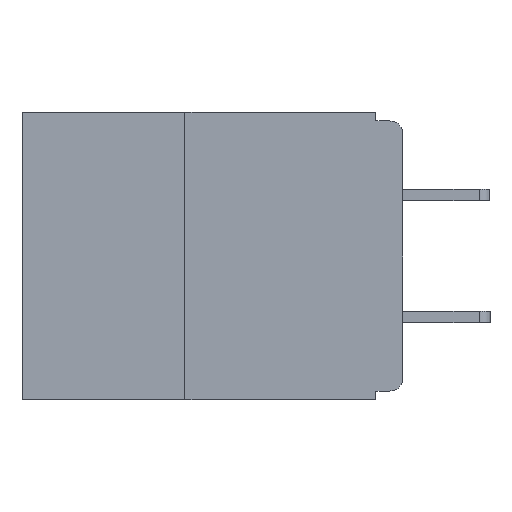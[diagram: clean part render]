
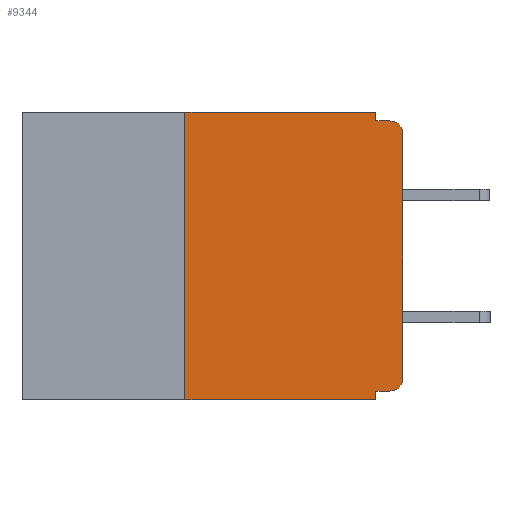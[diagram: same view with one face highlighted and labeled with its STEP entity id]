
A CAD part, left-side view. The second image highlights one B-rep face of the part: STEP entity #9344.
In plain terms, the highlighted planar face has unit normal (-1, 0, 0).
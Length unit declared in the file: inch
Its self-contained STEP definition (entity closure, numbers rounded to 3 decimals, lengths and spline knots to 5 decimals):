
#28 = CARTESIAN_POINT ( 'NONE',  ( 0., 0.031, -0.01 ) ) ;
#310 = VERTEX_POINT ( 'NONE', #12616 ) ;
#390 = CARTESIAN_POINT ( 'NONE',  ( 0., 0.437, -0.33 ) ) ;
#530 = CARTESIAN_POINT ( 'NONE',  ( 0., 0.015, -0.01 ) ) ;
#1196 = LINE ( 'NONE', #18396, #6299 ) ;
#1780 = VERTEX_POINT ( 'NONE', #16016 ) ;
#1913 = LINE ( 'NONE', #8565, #17554 ) ;
#2015 = VECTOR ( 'NONE', #24673, 39.37008 ) ;
#2554 = DIRECTION ( 'NONE',  ( 0., 1., 0. ) ) ;
#2694 = DIRECTION ( 'NONE',  ( 0., 0., -1. ) ) ;
#2735 = CARTESIAN_POINT ( 'NONE',  ( 0., 0.031, 0. ) ) ;
#2963 = DIRECTION ( 'NONE',  ( 0., 0., 1. ) ) ;
#4856 = VERTEX_POINT ( 'NONE', #12094 ) ;
#5527 = EDGE_CURVE ( 'NONE', #16227, #8673, #24029, .T. ) ;
#5559 = ORIENTED_EDGE ( 'NONE', *, *, #15498, .T. ) ;
#5974 = ORIENTED_EDGE ( 'NONE', *, *, #18405, .F. ) ;
#6143 = EDGE_CURVE ( 'NONE', #23200, #10950, #21404, .T. ) ;
#6175 = ORIENTED_EDGE ( 'NONE', *, *, #25741, .F. ) ;
#6299 = VECTOR ( 'NONE', #7874, 39.37008 ) ;
#7097 = AXIS2_PLACEMENT_3D ( 'NONE', #14998, #14834, #14744 ) ;
#7189 = DIRECTION ( 'NONE',  ( 0., 0., -1. ) ) ;
#7194 = DIRECTION ( 'NONE',  ( 1., 0., 0. ) ) ;
#7321 = PLANE ( 'NONE',  #12634 ) ;
#7811 = ORIENTED_EDGE ( 'NONE', *, *, #22973, .T. ) ;
#7874 = DIRECTION ( 'NONE',  ( 0., 0., -1. ) ) ;
#8022 = CARTESIAN_POINT ( 'NONE',  ( 0., 0., -0.305 ) ) ;
#8434 = LINE ( 'NONE', #18432, #2015 ) ;
#8565 = CARTESIAN_POINT ( 'NONE',  ( 0., 0.437, 0. ) ) ;
#8673 = VERTEX_POINT ( 'NONE', #28 ) ;
#9007 = CARTESIAN_POINT ( 'NONE',  ( 0., 0.437, 0. ) ) ;
#9344 = ADVANCED_FACE ( 'NONE', ( #17871 ), #7321, .F. ) ;
#9552 = VERTEX_POINT ( 'NONE', #530 ) ;
#10211 = ORIENTED_EDGE ( 'NONE', *, *, #11828, .T. ) ;
#10950 = VERTEX_POINT ( 'NONE', #8022 ) ;
#11035 = DIRECTION ( 'NONE',  ( 0., 0., -1. ) ) ;
#11062 = DIRECTION ( 'NONE',  ( -1., 0., 0. ) ) ;
#11097 = CARTESIAN_POINT ( 'NONE',  ( 0., 0.015, -0.025 ) ) ;
#11737 = VECTOR ( 'NONE', #2554, 39.37008 ) ;
#11783 = CARTESIAN_POINT ( 'NONE',  ( 0., 0.25, -0.33 ) ) ;
#11828 = EDGE_CURVE ( 'NONE', #18574, #9552, #18435, .T. ) ;
#12094 = CARTESIAN_POINT ( 'NONE',  ( 0., 0.031, -0.33 ) ) ;
#12475 = VECTOR ( 'NONE', #13873, 39.37008 ) ;
#12616 = CARTESIAN_POINT ( 'NONE',  ( 0., 0.25, 0. ) ) ;
#12634 = AXIS2_PLACEMENT_3D ( 'NONE', #9007, #7194, #7189 ) ;
#12752 = ORIENTED_EDGE ( 'NONE', *, *, #18807, .F. ) ;
#13133 = CARTESIAN_POINT ( 'NONE',  ( 0., 0.25, -0.33 ) ) ;
#13311 = CARTESIAN_POINT ( 'NONE',  ( 0., 0., -0.025 ) ) ;
#13329 = LINE ( 'NONE', #390, #24446 ) ;
#13720 = VECTOR ( 'NONE', #2963, 39.37008 ) ;
#13873 = DIRECTION ( 'NONE',  ( 0., 0., 1. ) ) ;
#13917 = CARTESIAN_POINT ( 'NONE',  ( 0., 0.015, -0.32 ) ) ;
#14736 = VERTEX_POINT ( 'NONE', #13133 ) ;
#14744 = DIRECTION ( 'NONE',  ( 0., 0., -1. ) ) ;
#14834 = DIRECTION ( 'NONE',  ( -1., 0., 0. ) ) ;
#14998 = CARTESIAN_POINT ( 'NONE',  ( 0., 0.015, -0.305 ) ) ;
#15117 = ORIENTED_EDGE ( 'NONE', *, *, #27100, .F. ) ;
#15298 = DIRECTION ( 'NONE',  ( 0., -1., 0. ) ) ;
#15498 = EDGE_CURVE ( 'NONE', #10950, #18574, #19975, .T. ) ;
#16016 = CARTESIAN_POINT ( 'NONE',  ( 0., 0.031, -0.32 ) ) ;
#16023 = EDGE_CURVE ( 'NONE', #23200, #1780, #22868, .T. ) ;
#16227 = VERTEX_POINT ( 'NONE', #22132 ) ;
#16884 = AXIS2_PLACEMENT_3D ( 'NONE', #11097, #11062, #11035 ) ;
#16911 = DIRECTION ( 'NONE',  ( 0., -1., 0. ) ) ;
#17554 = VECTOR ( 'NONE', #16911, 39.37008 ) ;
#17871 = FACE_OUTER_BOUND ( 'NONE', #24104, .T. ) ;
#18396 = CARTESIAN_POINT ( 'NONE',  ( 0., 0.031, -0.33 ) ) ;
#18405 = EDGE_CURVE ( 'NONE', #310, #16227, #1913, .T. ) ;
#18432 = CARTESIAN_POINT ( 'NONE',  ( 0., 0., -0.01 ) ) ;
#18435 = CIRCLE ( 'NONE', #16884, 0.015 ) ;
#18574 = VERTEX_POINT ( 'NONE', #13311 ) ;
#18740 = LINE ( 'NONE', #11783, #12475 ) ;
#18807 = EDGE_CURVE ( 'NONE', #1780, #4856, #1196, .T. ) ;
#19118 = ORIENTED_EDGE ( 'NONE', *, *, #16023, .F. ) ;
#19165 = VECTOR ( 'NONE', #2694, 39.37008 ) ;
#19975 = LINE ( 'NONE', #22076, #13720 ) ;
#21404 = CIRCLE ( 'NONE', #7097, 0.015 ) ;
#22076 = CARTESIAN_POINT ( 'NONE',  ( 0., 0., 0. ) ) ;
#22132 = CARTESIAN_POINT ( 'NONE',  ( 0., 0.031, 0. ) ) ;
#22787 = ORIENTED_EDGE ( 'NONE', *, *, #6143, .T. ) ;
#22868 = LINE ( 'NONE', #25672, #11737 ) ;
#22973 = EDGE_CURVE ( 'NONE', #14736, #4856, #13329, .T. ) ;
#23200 = VERTEX_POINT ( 'NONE', #13917 ) ;
#24029 = LINE ( 'NONE', #2735, #19165 ) ;
#24104 = EDGE_LOOP ( 'NONE', ( #5559, #10211, #15117, #26339, #5974, #6175, #7811, #12752, #19118, #22787 ) ) ;
#24446 = VECTOR ( 'NONE', #15298, 39.37008 ) ;
#24673 = DIRECTION ( 'NONE',  ( 0., -1., 0. ) ) ;
#25672 = CARTESIAN_POINT ( 'NONE',  ( 0., 0., -0.32 ) ) ;
#25741 = EDGE_CURVE ( 'NONE', #14736, #310, #18740, .T. ) ;
#26339 = ORIENTED_EDGE ( 'NONE', *, *, #5527, .F. ) ;
#27100 = EDGE_CURVE ( 'NONE', #8673, #9552, #8434, .T. ) ;
